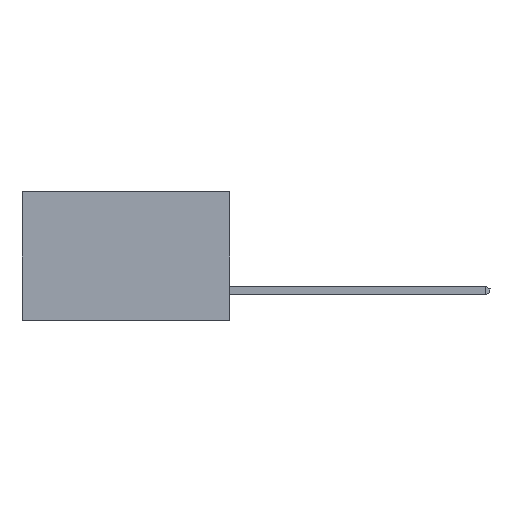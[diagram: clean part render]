
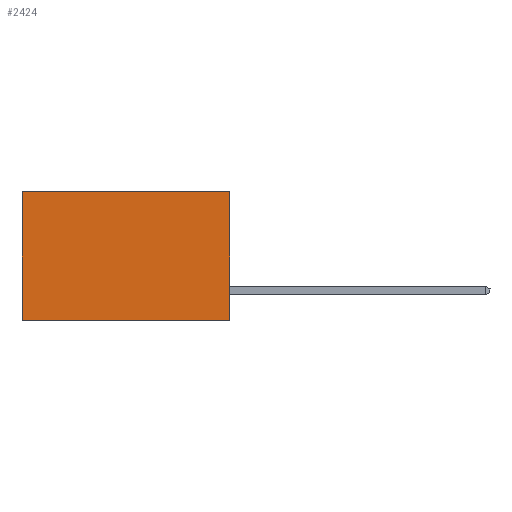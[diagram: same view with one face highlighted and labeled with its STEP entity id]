
A CAD part, left-side view. The second image highlights one B-rep face of the part: STEP entity #2424.
In plain terms, the highlighted planar face has unit normal (-1, 0, 0).
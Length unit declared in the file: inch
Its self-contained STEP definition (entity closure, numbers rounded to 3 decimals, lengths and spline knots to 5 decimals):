
#370 = CARTESIAN_POINT ( 'NONE',  ( 0.2615, 0., -0.37 ) ) ;
#544 = DIRECTION ( 'NONE',  ( 0., 0., -1. ) ) ;
#757 = VERTEX_POINT ( 'NONE', #370 ) ;
#2424 = ADVANCED_FACE ( 'NONE', ( #13515 ), #20317, .F. ) ;
#4629 = VERTEX_POINT ( 'NONE', #10889 ) ;
#5892 = DIRECTION ( 'NONE',  ( 0., 1., 0. ) ) ;
#5946 = LINE ( 'NONE', #15909, #20831 ) ;
#6320 = LINE ( 'NONE', #16397, #19411 ) ;
#6541 = EDGE_CURVE ( 'NONE', #20033, #4629, #17311, .T. ) ;
#7034 = ORIENTED_EDGE ( 'NONE', *, *, #17753, .F. ) ;
#7085 = CARTESIAN_POINT ( 'NONE',  ( 0.2615, 0., -0.37 ) ) ;
#7381 = ORIENTED_EDGE ( 'NONE', *, *, #6541, .T. ) ;
#7749 = DIRECTION ( 'NONE',  ( 0., 0., -1. ) ) ;
#8533 = CARTESIAN_POINT ( 'NONE',  ( 0.2615, 0., -0.37 ) ) ;
#8727 = DIRECTION ( 'NONE',  ( 1., 0., 0. ) ) ;
#8752 = AXIS2_PLACEMENT_3D ( 'NONE', #7085, #8727, #15491 ) ;
#8880 = CARTESIAN_POINT ( 'NONE',  ( 0.2615, 0., 0. ) ) ;
#9979 = DIRECTION ( 'NONE',  ( 0., 1., 0. ) ) ;
#10692 = VERTEX_POINT ( 'NONE', #17161 ) ;
#10889 = CARTESIAN_POINT ( 'NONE',  ( 0.2615, 0.6, 0. ) ) ;
#13306 = LINE ( 'NONE', #8533, #16170 ) ;
#13515 = FACE_OUTER_BOUND ( 'NONE', #14552, .T. ) ;
#14552 = EDGE_LOOP ( 'NONE', ( #20279, #7034, #21133, #7381 ) ) ;
#15491 = DIRECTION ( 'NONE',  ( 0., 0., -1. ) ) ;
#15909 = CARTESIAN_POINT ( 'NONE',  ( 0.2615, 0., -0.37 ) ) ;
#16170 = VECTOR ( 'NONE', #9979, 39.37008 ) ;
#16397 = CARTESIAN_POINT ( 'NONE',  ( 0.2615, 0.6, -0.37 ) ) ;
#17161 = CARTESIAN_POINT ( 'NONE',  ( 0.2615, 0.6, -0.37 ) ) ;
#17311 = LINE ( 'NONE', #8880, #19544 ) ;
#17753 = EDGE_CURVE ( 'NONE', #757, #10692, #13306, .T. ) ;
#18078 = EDGE_CURVE ( 'NONE', #4629, #10692, #6320, .T. ) ;
#18153 = CARTESIAN_POINT ( 'NONE',  ( 0.2615, 0., 0. ) ) ;
#19411 = VECTOR ( 'NONE', #7749, 39.37008 ) ;
#19544 = VECTOR ( 'NONE', #5892, 39.37008 ) ;
#19888 = EDGE_CURVE ( 'NONE', #20033, #757, #5946, .T. ) ;
#20033 = VERTEX_POINT ( 'NONE', #18153 ) ;
#20279 = ORIENTED_EDGE ( 'NONE', *, *, #18078, .T. ) ;
#20317 = PLANE ( 'NONE',  #8752 ) ;
#20831 = VECTOR ( 'NONE', #544, 39.37008 ) ;
#21133 = ORIENTED_EDGE ( 'NONE', *, *, #19888, .F. ) ;
